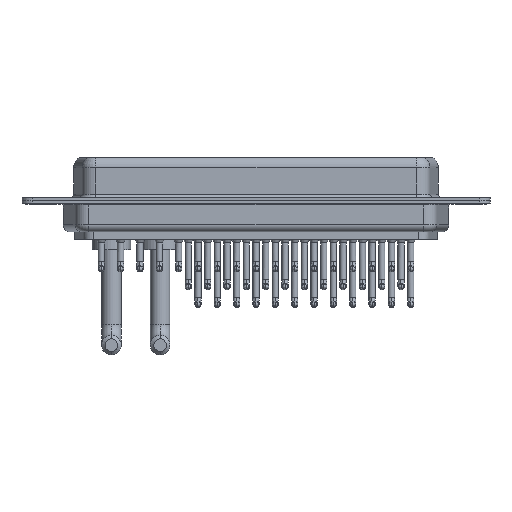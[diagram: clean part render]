
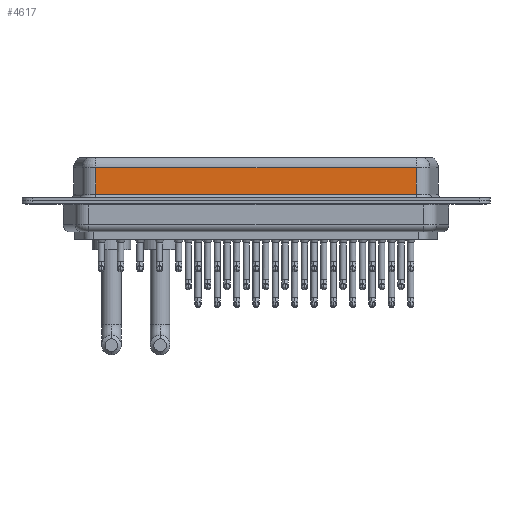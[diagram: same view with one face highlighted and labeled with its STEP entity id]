
A CAD part, front view. The second image highlights one B-rep face of the part: STEP entity #4617.
In plain terms, the highlighted planar face has unit normal (0, -1, 0).
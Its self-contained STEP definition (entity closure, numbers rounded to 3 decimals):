
#413 = CARTESIAN_POINT ( 'NONE',  ( 7.59, -5.375, 0.9 ) ) ;
#1161 = LINE ( 'NONE', #10645, #6715 ) ;
#1244 = EDGE_CURVE ( 'NONE', #26364, #15224, #6539, .T. ) ;
#4092 = PLANE ( 'NONE',  #14792 ) ;
#4617 = ADVANCED_FACE ( 'NONE', ( #6570 ), #4092, .F. ) ;
#4842 = CARTESIAN_POINT ( 'NONE',  ( 53.41, -5.375, 6.4 ) ) ;
#5497 = ORIENTED_EDGE ( 'NONE', *, *, #5631, .T. ) ;
#5631 = EDGE_CURVE ( 'NONE', #10610, #28812, #30607, .T. ) ;
#5755 = VECTOR ( 'NONE', #28738, 1000. ) ;
#6495 = CARTESIAN_POINT ( 'NONE',  ( 53.41, -5.375, 0.9 ) ) ;
#6539 = LINE ( 'NONE', #29709, #9604 ) ;
#6570 = FACE_OUTER_BOUND ( 'NONE', #7779, .T. ) ;
#6715 = VECTOR ( 'NONE', #20118, 1000. ) ;
#7779 = EDGE_LOOP ( 'NONE', ( #24757, #5497, #21728, #7945 ) ) ;
#7945 = ORIENTED_EDGE ( 'NONE', *, *, #1244, .T. ) ;
#9604 = VECTOR ( 'NONE', #13378, 1000. ) ;
#10610 = VERTEX_POINT ( 'NONE', #12756 ) ;
#10645 = CARTESIAN_POINT ( 'NONE',  ( 7.59, -5.375, 6.4 ) ) ;
#12756 = CARTESIAN_POINT ( 'NONE',  ( 53.41, -5.375, 4.65 ) ) ;
#13378 = DIRECTION ( 'NONE',  ( 1., 0., 0. ) ) ;
#14149 = EDGE_CURVE ( 'NONE', #28812, #26364, #1161, .T. ) ;
#14304 = DIRECTION ( 'NONE',  ( 0., 0., -1. ) ) ;
#14792 = AXIS2_PLACEMENT_3D ( 'NONE', #18240, #29904, #18546 ) ;
#15224 = VERTEX_POINT ( 'NONE', #6495 ) ;
#16289 = CARTESIAN_POINT ( 'NONE',  ( 53.41, -5.375, 4.65 ) ) ;
#16951 = LINE ( 'NONE', #4842, #17721 ) ;
#17721 = VECTOR ( 'NONE', #14304, 1000. ) ;
#18240 = CARTESIAN_POINT ( 'NONE',  ( 53.41, -5.375, 6.4 ) ) ;
#18546 = DIRECTION ( 'NONE',  ( 0., 0., 1. ) ) ;
#20118 = DIRECTION ( 'NONE',  ( 0., 0., -1. ) ) ;
#21096 = CARTESIAN_POINT ( 'NONE',  ( 7.59, -5.375, 4.65 ) ) ;
#21728 = ORIENTED_EDGE ( 'NONE', *, *, #14149, .T. ) ;
#24757 = ORIENTED_EDGE ( 'NONE', *, *, #25559, .F. ) ;
#25559 = EDGE_CURVE ( 'NONE', #10610, #15224, #16951, .T. ) ;
#26364 = VERTEX_POINT ( 'NONE', #413 ) ;
#28738 = DIRECTION ( 'NONE',  ( -1., 0., 0. ) ) ;
#28812 = VERTEX_POINT ( 'NONE', #21096 ) ;
#29709 = CARTESIAN_POINT ( 'NONE',  ( 53.41, -5.375, 0.9 ) ) ;
#29904 = DIRECTION ( 'NONE',  ( 0., 1., 0. ) ) ;
#30607 = LINE ( 'NONE', #16289, #5755 ) ;
